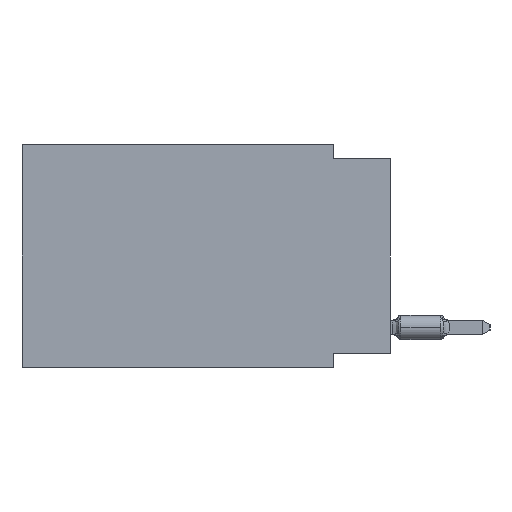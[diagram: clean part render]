
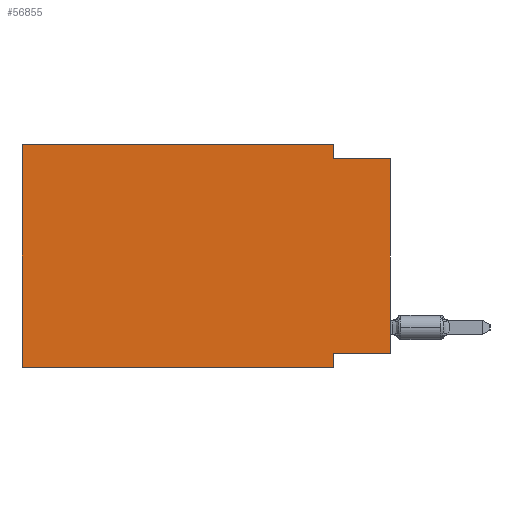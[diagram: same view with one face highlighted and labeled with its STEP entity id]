
A CAD part, left-side view. The second image highlights one B-rep face of the part: STEP entity #56855.
In plain terms, the highlighted planar face has unit normal (-1, 0, 0).
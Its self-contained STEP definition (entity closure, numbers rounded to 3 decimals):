
#334 = DIRECTION ( 'NONE',  ( 0., 0., -1. ) ) ;
#814 = VERTEX_POINT ( 'NONE', #28360 ) ;
#1052 = VECTOR ( 'NONE', #20500, 1000. ) ;
#2355 = ORIENTED_EDGE ( 'NONE', *, *, #36611, .T. ) ;
#2760 = EDGE_CURVE ( 'NONE', #814, #52129, #30474, .T. ) ;
#3532 = VERTEX_POINT ( 'NONE', #42374 ) ;
#3778 = VECTOR ( 'NONE', #16225, 1000. ) ;
#4306 = VERTEX_POINT ( 'NONE', #22317 ) ;
#4991 = LINE ( 'NONE', #23731, #3778 ) ;
#6579 = VECTOR ( 'NONE', #12474, 1000. ) ;
#6667 = CARTESIAN_POINT ( 'NONE',  ( 0., 0., 0. ) ) ;
#6746 = LINE ( 'NONE', #21468, #36416 ) ;
#11276 = DIRECTION ( 'NONE',  ( 0., 0., -1. ) ) ;
#12474 = DIRECTION ( 'NONE',  ( 0., -1., 0. ) ) ;
#16225 = DIRECTION ( 'NONE',  ( 0., -1., 0. ) ) ;
#16522 = DIRECTION ( 'NONE',  ( 0., 0., -1. ) ) ;
#18364 = CARTESIAN_POINT ( 'NONE',  ( 0., 2.54, -9.906 ) ) ;
#18790 = VERTEX_POINT ( 'NONE', #18364 ) ;
#19966 = EDGE_CURVE ( 'NONE', #52129, #18790, #28257, .T. ) ;
#20033 = EDGE_CURVE ( 'NONE', #3532, #21813, #6746, .T. ) ;
#20500 = DIRECTION ( 'NONE',  ( 0., 0., 1. ) ) ;
#21468 = CARTESIAN_POINT ( 'NONE',  ( 0., 16.383, 0. ) ) ;
#21813 = VERTEX_POINT ( 'NONE', #53059 ) ;
#22317 = CARTESIAN_POINT ( 'NONE',  ( 0., 2.54, -0.635 ) ) ;
#23666 = CARTESIAN_POINT ( 'NONE',  ( 0., 2.54, -9.906 ) ) ;
#23731 = CARTESIAN_POINT ( 'NONE',  ( 0., 0., -0.635 ) ) ;
#24810 = PLANE ( 'NONE',  #58054 ) ;
#26185 = VECTOR ( 'NONE', #16522, 1000. ) ;
#27108 = VECTOR ( 'NONE', #35396, 1000. ) ;
#27256 = ORIENTED_EDGE ( 'NONE', *, *, #2760, .F. ) ;
#28210 = EDGE_CURVE ( 'NONE', #56014, #4306, #54030, .T. ) ;
#28257 = LINE ( 'NONE', #23666, #55033 ) ;
#28360 = CARTESIAN_POINT ( 'NONE',  ( 0., 0., -9.271 ) ) ;
#28451 = VERTEX_POINT ( 'NONE', #32493 ) ;
#28565 = ORIENTED_EDGE ( 'NONE', *, *, #28210, .F. ) ;
#30474 = LINE ( 'NONE', #58419, #27108 ) ;
#31378 = EDGE_CURVE ( 'NONE', #4306, #28451, #4991, .T. ) ;
#31839 = ORIENTED_EDGE ( 'NONE', *, *, #43841, .F. ) ;
#32493 = CARTESIAN_POINT ( 'NONE',  ( 0., 0., -0.635 ) ) ;
#34289 = LINE ( 'NONE', #38897, #36614 ) ;
#34556 = CARTESIAN_POINT ( 'NONE',  ( 0., 2.54, 0. ) ) ;
#35396 = DIRECTION ( 'NONE',  ( 0., 1., 0. ) ) ;
#36416 = VECTOR ( 'NONE', #40215, 1000. ) ;
#36611 = EDGE_CURVE ( 'NONE', #3532, #18790, #34289, .T. ) ;
#36614 = VECTOR ( 'NONE', #53023, 1000. ) ;
#38897 = CARTESIAN_POINT ( 'NONE',  ( 0., 16.383, -9.906 ) ) ;
#40174 = EDGE_LOOP ( 'NONE', ( #40508, #44937, #28565, #31839, #52488, #2355, #57331, #27256 ) ) ;
#40215 = DIRECTION ( 'NONE',  ( 0., 0., 1. ) ) ;
#40508 = ORIENTED_EDGE ( 'NONE', *, *, #55618, .T. ) ;
#40559 = CARTESIAN_POINT ( 'NONE',  ( 0., 2.54, -9.271 ) ) ;
#42374 = CARTESIAN_POINT ( 'NONE',  ( 0., 16.383, -9.906 ) ) ;
#43568 = DIRECTION ( 'NONE',  ( 1., 0., 0. ) ) ;
#43633 = CARTESIAN_POINT ( 'NONE',  ( 0., 2.54, 0. ) ) ;
#43841 = EDGE_CURVE ( 'NONE', #21813, #56014, #54274, .T. ) ;
#44147 = LINE ( 'NONE', #6667, #1052 ) ;
#44937 = ORIENTED_EDGE ( 'NONE', *, *, #31378, .F. ) ;
#49359 = FACE_OUTER_BOUND ( 'NONE', #40174, .T. ) ;
#52129 = VERTEX_POINT ( 'NONE', #40559 ) ;
#52488 = ORIENTED_EDGE ( 'NONE', *, *, #20033, .F. ) ;
#53023 = DIRECTION ( 'NONE',  ( 0., -1., 0. ) ) ;
#53059 = CARTESIAN_POINT ( 'NONE',  ( 0., 16.383, 0. ) ) ;
#54030 = LINE ( 'NONE', #43633, #26185 ) ;
#54274 = LINE ( 'NONE', #54869, #6579 ) ;
#54869 = CARTESIAN_POINT ( 'NONE',  ( 0., 16.383, 0. ) ) ;
#55033 = VECTOR ( 'NONE', #334, 1000. ) ;
#55618 = EDGE_CURVE ( 'NONE', #814, #28451, #44147, .T. ) ;
#56014 = VERTEX_POINT ( 'NONE', #34556 ) ;
#56855 = ADVANCED_FACE ( 'NONE', ( #49359 ), #24810, .F. ) ;
#57331 = ORIENTED_EDGE ( 'NONE', *, *, #19966, .F. ) ;
#57966 = CARTESIAN_POINT ( 'NONE',  ( 0., 16.383, 0. ) ) ;
#58054 = AXIS2_PLACEMENT_3D ( 'NONE', #57966, #43568, #11276 ) ;
#58419 = CARTESIAN_POINT ( 'NONE',  ( 0., 0., -9.271 ) ) ;
